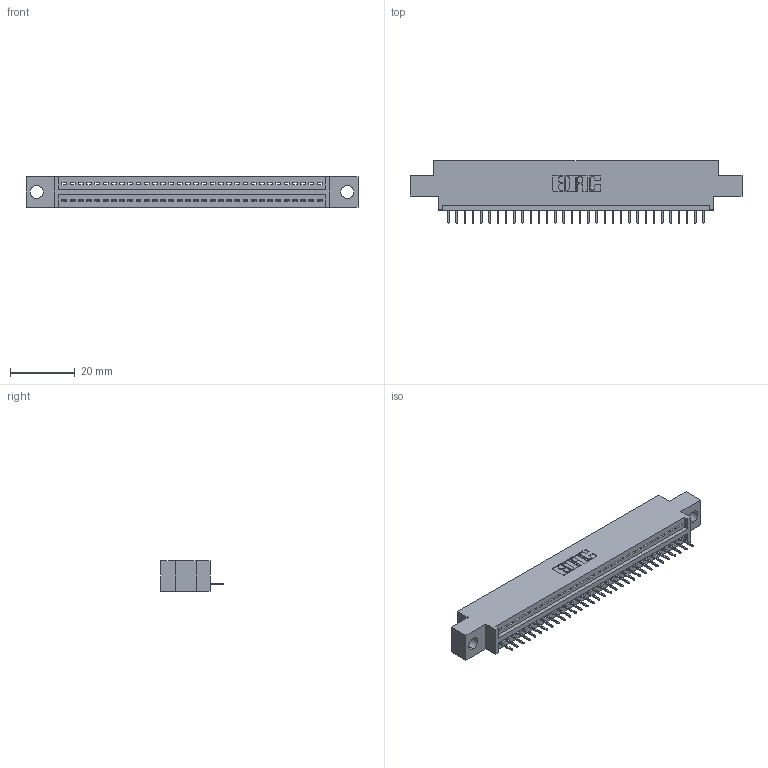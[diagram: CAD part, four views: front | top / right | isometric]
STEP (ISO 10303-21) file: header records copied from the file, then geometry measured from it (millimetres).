
FILE_DESCRIPTION (( 'STEP AP203' ), '1' );
FILE_NAME ('345-032-524-604.STEP', '2021-05-26T14:42:15', ( '' ), ( '' ), 'SwSTEP 2.0', 'SolidWorks 2020', '' );
FILE_SCHEMA (( 'CONFIG_CONTROL_DESIGN' ));
Length unit declared in the file: inch
Products named in the file (3): 345-292-001_345-293-124; 345-032-524-604; 345 Part_0.170 Offset - 0.156 Dia-TI
Assembly tree (33 placements, depth 2):
  345-032-524-604
    345 Part_0.170 Offset - 0.156 Dia-TI
    345-292-001_345-293-124  x32
Bounding box: 102.49 x 19.35 x 9.4 mm (x, y, z)
Volume: 9306.9 mm3; surface area: 11796.9 mm2
Topology: 33 solids, 33 shells, 2128 faces, 6149 edges, 3970 vertices
Faces by surface type: plane 1570, cylinder 558
Entity records: 26055 total; most frequent: CARTESIAN_POINT 4522, ORIENTED_EDGE 4486, DIRECTION 3963, EDGE_CURVE 2243, LINE 1987, VECTOR 1987, VERTEX_POINT 1490, AXIS2_PLACEMENT_3D 988
